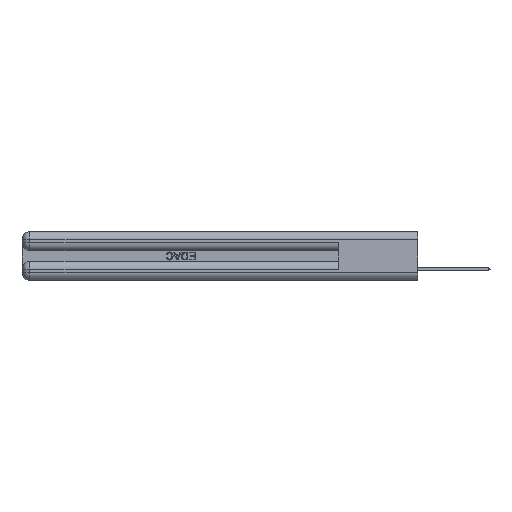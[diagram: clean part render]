
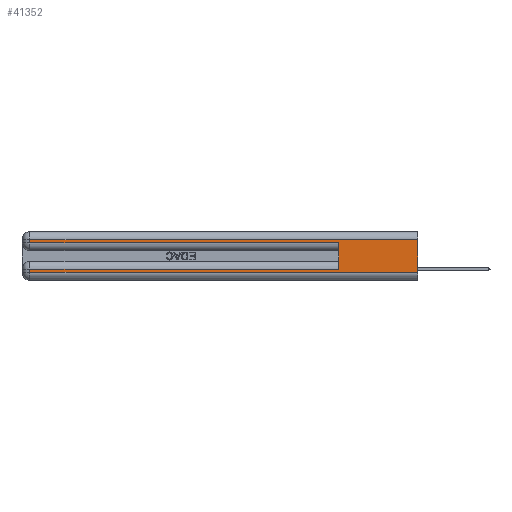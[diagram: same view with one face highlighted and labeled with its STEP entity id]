
A CAD part, left-side view. The second image highlights one B-rep face of the part: STEP entity #41352.
In plain terms, the highlighted planar face has unit normal (-1, 0, 0).
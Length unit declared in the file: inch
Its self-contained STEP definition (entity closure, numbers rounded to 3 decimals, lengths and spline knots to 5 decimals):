
#12 = VERTEX_POINT ( 'NONE', #10869 ) ;
#296 = CARTESIAN_POINT ( 'NONE',  ( 0., 0., 0.085 ) ) ;
#918 = LINE ( 'NONE', #27986, #35642 ) ;
#1279 = EDGE_CURVE ( 'NONE', #17511, #41393, #3366, .T. ) ;
#3366 = LINE ( 'NONE', #4143, #27598 ) ;
#4044 = EDGE_CURVE ( 'NONE', #43391, #15995, #918, .T. ) ;
#4143 = CARTESIAN_POINT ( 'NONE',  ( 0., 0.6, 0.145 ) ) ;
#5162 = ORIENTED_EDGE ( 'NONE', *, *, #1279, .F. ) ;
#6029 = VECTOR ( 'NONE', #27637, 39.37008 ) ;
#6316 = ORIENTED_EDGE ( 'NONE', *, *, #37569, .F. ) ;
#6790 = CARTESIAN_POINT ( 'NONE',  ( 0., 0., 0.37 ) ) ;
#6934 = CARTESIAN_POINT ( 'NONE',  ( 0., 0.6, 0.285 ) ) ;
#9661 = EDGE_CURVE ( 'NONE', #33190, #41393, #35857, .T. ) ;
#10825 = CARTESIAN_POINT ( 'NONE',  ( 0., 2.94, 0.085 ) ) ;
#10869 = CARTESIAN_POINT ( 'NONE',  ( 0., 2.94, 0.31 ) ) ;
#11311 = AXIS2_PLACEMENT_3D ( 'NONE', #6790, #36636, #26562 ) ;
#12761 = CARTESIAN_POINT ( 'NONE',  ( 0., 0., 0.06 ) ) ;
#13364 = CARTESIAN_POINT ( 'NONE',  ( 0., 0., 0.285 ) ) ;
#13371 = VECTOR ( 'NONE', #23322, 39.37008 ) ;
#14073 = VECTOR ( 'NONE', #17913, 39.37008 ) ;
#14082 = ORIENTED_EDGE ( 'NONE', *, *, #40341, .T. ) ;
#15995 = VERTEX_POINT ( 'NONE', #24333 ) ;
#16942 = CARTESIAN_POINT ( 'NONE',  ( 0., 0., 0.31 ) ) ;
#17350 = ORIENTED_EDGE ( 'NONE', *, *, #9661, .T. ) ;
#17438 = FACE_OUTER_BOUND ( 'NONE', #34398, .T. ) ;
#17452 = EDGE_CURVE ( 'NONE', #15995, #18709, #18641, .T. ) ;
#17511 = VERTEX_POINT ( 'NONE', #25252 ) ;
#17913 = DIRECTION ( 'NONE',  ( 0., 0., -1. ) ) ;
#18641 = LINE ( 'NONE', #41175, #6029 ) ;
#18709 = VERTEX_POINT ( 'NONE', #12761 ) ;
#23087 = LINE ( 'NONE', #34775, #14073 ) ;
#23322 = DIRECTION ( 'NONE',  ( 0., 1., 0. ) ) ;
#23477 = PLANE ( 'NONE',  #11311 ) ;
#23639 = CARTESIAN_POINT ( 'NONE',  ( 0., 0., 0.37 ) ) ;
#23716 = LINE ( 'NONE', #29393, #35757 ) ;
#23974 = DIRECTION ( 'NONE',  ( 0., -1., 0. ) ) ;
#24333 = CARTESIAN_POINT ( 'NONE',  ( 0., 2.94, 0.06 ) ) ;
#25050 = ORIENTED_EDGE ( 'NONE', *, *, #17452, .T. ) ;
#25252 = CARTESIAN_POINT ( 'NONE',  ( 0., 0.6, 0.085 ) ) ;
#26562 = DIRECTION ( 'NONE',  ( 0., 0., -1. ) ) ;
#27598 = VECTOR ( 'NONE', #37922, 39.37008 ) ;
#27637 = DIRECTION ( 'NONE',  ( 0., -1., 0. ) ) ;
#27986 = CARTESIAN_POINT ( 'NONE',  ( 0., 2.94, 0.37 ) ) ;
#28924 = ORIENTED_EDGE ( 'NONE', *, *, #29243, .T. ) ;
#29243 = EDGE_CURVE ( 'NONE', #38643, #12, #23716, .T. ) ;
#29393 = CARTESIAN_POINT ( 'NONE',  ( 0., 0., 0.31 ) ) ;
#31154 = ORIENTED_EDGE ( 'NONE', *, *, #4044, .T. ) ;
#31863 = CARTESIAN_POINT ( 'NONE',  ( 0., 2.94, 0.285 ) ) ;
#32074 = ORIENTED_EDGE ( 'NONE', *, *, #34113, .T. ) ;
#32492 = VECTOR ( 'NONE', #33849, 39.37008 ) ;
#33190 = VERTEX_POINT ( 'NONE', #31863 ) ;
#33849 = DIRECTION ( 'NONE',  ( 0., 0., -1. ) ) ;
#34113 = EDGE_CURVE ( 'NONE', #17511, #43391, #43385, .T. ) ;
#34398 = EDGE_LOOP ( 'NONE', ( #6316, #28924, #14082, #17350, #5162, #32074, #31154, #25050 ) ) ;
#34775 = CARTESIAN_POINT ( 'NONE',  ( 0., 2.94, 0.37 ) ) ;
#35281 = DIRECTION ( 'NONE',  ( 0., 0., -1. ) ) ;
#35642 = VECTOR ( 'NONE', #35281, 39.37008 ) ;
#35757 = VECTOR ( 'NONE', #42660, 39.37008 ) ;
#35857 = LINE ( 'NONE', #13364, #39543 ) ;
#36636 = DIRECTION ( 'NONE',  ( 1., 0., 0. ) ) ;
#37190 = LINE ( 'NONE', #23639, #32492 ) ;
#37569 = EDGE_CURVE ( 'NONE', #38643, #18709, #37190, .T. ) ;
#37922 = DIRECTION ( 'NONE',  ( 0., 0., 1. ) ) ;
#38643 = VERTEX_POINT ( 'NONE', #16942 ) ;
#39543 = VECTOR ( 'NONE', #23974, 39.37008 ) ;
#40341 = EDGE_CURVE ( 'NONE', #12, #33190, #23087, .T. ) ;
#41175 = CARTESIAN_POINT ( 'NONE',  ( 0., 0., 0.06 ) ) ;
#41352 = ADVANCED_FACE ( 'NONE', ( #17438 ), #23477, .F. ) ;
#41393 = VERTEX_POINT ( 'NONE', #6934 ) ;
#42660 = DIRECTION ( 'NONE',  ( 0., 1., 0. ) ) ;
#43385 = LINE ( 'NONE', #296, #13371 ) ;
#43391 = VERTEX_POINT ( 'NONE', #10825 ) ;
